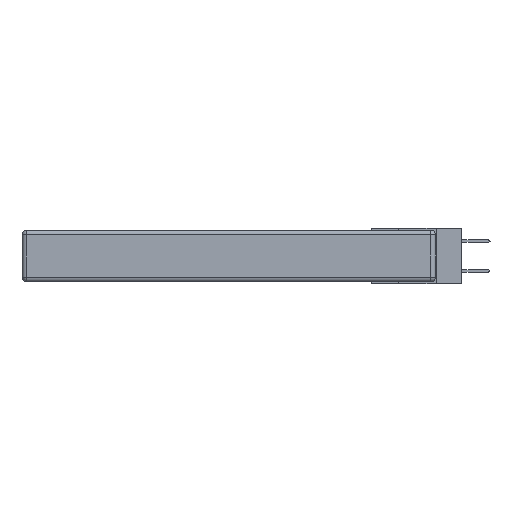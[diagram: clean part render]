
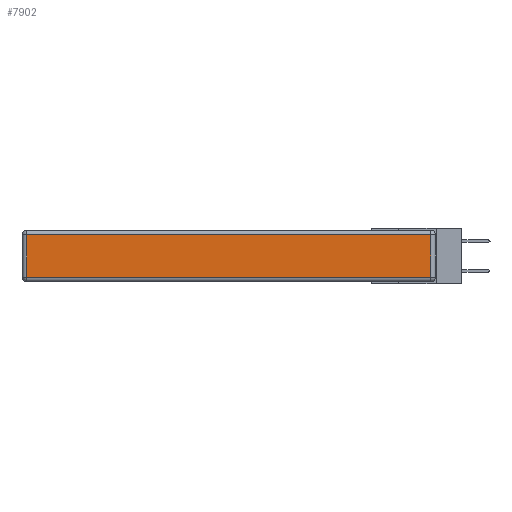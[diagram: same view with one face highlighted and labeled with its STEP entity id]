
A CAD part, left-side view. The second image highlights one B-rep face of the part: STEP entity #7902.
In plain terms, the highlighted planar face has unit normal (-1, 0, 0).
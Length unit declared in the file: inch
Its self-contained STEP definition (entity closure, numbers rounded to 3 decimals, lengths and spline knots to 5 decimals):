
#263 = ORIENTED_EDGE ( 'NONE', *, *, #12749, .T. ) ;
#923 = VERTEX_POINT ( 'NONE', #7287 ) ;
#999 = CARTESIAN_POINT ( 'NONE',  ( 0., 0.03, -0.03 ) ) ;
#1161 = VECTOR ( 'NONE', #15494, 39.37008 ) ;
#1642 = AXIS2_PLACEMENT_3D ( 'NONE', #13539, #9954, #6373 ) ;
#2233 = CARTESIAN_POINT ( 'NONE',  ( 0., 0.03, -0.343 ) ) ;
#2387 = LINE ( 'NONE', #10822, #9540 ) ;
#2566 = EDGE_CURVE ( 'NONE', #10977, #923, #2387, .T. ) ;
#2836 = EDGE_CURVE ( 'NONE', #12021, #10977, #4059, .T. ) ;
#3141 = EDGE_CURVE ( 'NONE', #923, #15040, #10649, .T. ) ;
#3239 = ORIENTED_EDGE ( 'NONE', *, *, #2836, .T. ) ;
#3279 = CARTESIAN_POINT ( 'NONE',  ( 0., 2.72, -0.03 ) ) ;
#4059 = LINE ( 'NONE', #14159, #14793 ) ;
#4207 = ORIENTED_EDGE ( 'NONE', *, *, #3141, .T. ) ;
#4289 = EDGE_LOOP ( 'NONE', ( #4207, #263, #3239, #4727 ) ) ;
#4618 = CARTESIAN_POINT ( 'NONE',  ( 0., 0.03, -0.313 ) ) ;
#4727 = ORIENTED_EDGE ( 'NONE', *, *, #2566, .T. ) ;
#5132 = PLANE ( 'NONE',  #1642 ) ;
#6004 = CARTESIAN_POINT ( 'NONE',  ( 0., 0., -0.313 ) ) ;
#6373 = DIRECTION ( 'NONE',  ( 0., 0., 1. ) ) ;
#7287 = CARTESIAN_POINT ( 'NONE',  ( 0., 2.72, -0.313 ) ) ;
#7902 = ADVANCED_FACE ( 'NONE', ( #11526 ), #5132, .T. ) ;
#9540 = VECTOR ( 'NONE', #13143, 39.37008 ) ;
#9654 = DIRECTION ( 'NONE',  ( 0., -1., 0. ) ) ;
#9885 = VECTOR ( 'NONE', #9654, 39.37008 ) ;
#9954 = DIRECTION ( 'NONE',  ( -1., 0., 0. ) ) ;
#10649 = LINE ( 'NONE', #6004, #9885 ) ;
#10822 = CARTESIAN_POINT ( 'NONE',  ( 0., 2.72, -0.343 ) ) ;
#10977 = VERTEX_POINT ( 'NONE', #3279 ) ;
#11526 = FACE_OUTER_BOUND ( 'NONE', #4289, .T. ) ;
#12021 = VERTEX_POINT ( 'NONE', #999 ) ;
#12749 = EDGE_CURVE ( 'NONE', #15040, #12021, #13372, .T. ) ;
#12777 = DIRECTION ( 'NONE',  ( 0., 1., 0. ) ) ;
#13143 = DIRECTION ( 'NONE',  ( 0., 0., -1. ) ) ;
#13372 = LINE ( 'NONE', #2233, #1161 ) ;
#13539 = CARTESIAN_POINT ( 'NONE',  ( 0., 0., -0.343 ) ) ;
#14159 = CARTESIAN_POINT ( 'NONE',  ( 0., 2.75, -0.03 ) ) ;
#14793 = VECTOR ( 'NONE', #12777, 39.37008 ) ;
#15040 = VERTEX_POINT ( 'NONE', #4618 ) ;
#15494 = DIRECTION ( 'NONE',  ( 0., 0., 1. ) ) ;
